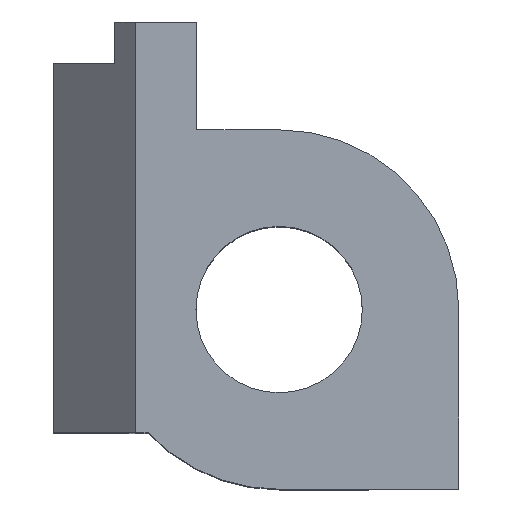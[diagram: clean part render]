
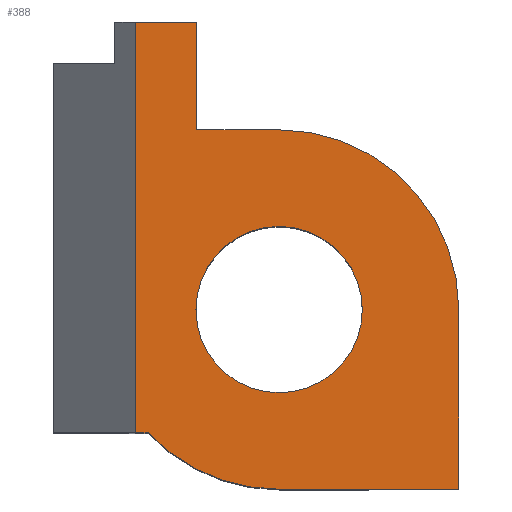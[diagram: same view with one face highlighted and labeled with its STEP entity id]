
A CAD part, top view. The second image highlights one B-rep face of the part: STEP entity #388.
In plain terms, the highlighted planar face has unit normal (0, 0, 1).
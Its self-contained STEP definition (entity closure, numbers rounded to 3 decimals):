
#222=CARTESIAN_POINT('',(-7.,14.,9.9));
#223=VERTEX_POINT('',#222);
#230=CARTESIAN_POINT('',(-4.,14.,9.9));
#231=VERTEX_POINT('',#230);
#232=CARTESIAN_POINT('',(-7.,14.,9.9));
#233=DIRECTION('',(1.0,0.0,0.0));
#234=VECTOR('',#233,3.);
#235=LINE('',#232,#234);
#236=EDGE_CURVE('',#223,#231,#235,.T.);
#293=CARTESIAN_POINT('',(-7.,-6.,9.9));
#294=VERTEX_POINT('',#293);
#301=CARTESIAN_POINT('',(-7.,-6.,9.9));
#302=DIRECTION('',(0.0,1.0,0.0));
#303=VECTOR('',#302,20.);
#304=LINE('',#301,#303);
#305=EDGE_CURVE('',#294,#223,#304,.T.);
#312=CARTESIAN_POINT('',(-9.5,13.0,9.9));
#313=DIRECTION('',(0.0,0.0,1.0));
#314=DIRECTION('',(1.0,0.0,0.0));
#315=AXIS2_PLACEMENT_3D('',#312,#313,#314);
#316=PLANE('',#315);
#317=ORIENTED_EDGE('',*,*,#305,.F.);
#318=CARTESIAN_POINT('',(-6.369,-6.,9.9));
#319=VERTEX_POINT('',#318);
#320=CARTESIAN_POINT('',(-6.369,-6.,9.9));
#321=DIRECTION('',(-1.0,0.0,0.0));
#322=VECTOR('',#321,0.631);
#323=LINE('',#320,#322);
#324=EDGE_CURVE('',#319,#294,#323,.T.);
#325=ORIENTED_EDGE('',*,*,#324,.F.);
#326=CARTESIAN_POINT('',(0.,-8.75,9.9));
#327=VERTEX_POINT('',#326);
#328=CARTESIAN_POINT('',(0.0,0.0,9.9));
#329=DIRECTION('',(0.0,0.0,-1.0));
#330=DIRECTION('',(1.0,0.0,0.0));
#331=AXIS2_PLACEMENT_3D('',#328,#329,#330);
#332=CIRCLE('',#331,8.75);
#333=EDGE_CURVE('',#327,#319,#332,.T.);
#334=ORIENTED_EDGE('',*,*,#333,.F.);
#335=CARTESIAN_POINT('',(8.75,-8.75,9.9));
#336=VERTEX_POINT('',#335);
#337=CARTESIAN_POINT('',(8.75,-8.75,9.9));
#338=DIRECTION('',(-1.0,0.0,0.0));
#339=VECTOR('',#338,8.75);
#340=LINE('',#337,#339);
#341=EDGE_CURVE('',#336,#327,#340,.T.);
#342=ORIENTED_EDGE('',*,*,#341,.F.);
#343=CARTESIAN_POINT('',(8.75,0.,9.9));
#344=VERTEX_POINT('',#343);
#345=CARTESIAN_POINT('',(8.75,0.,9.9));
#346=DIRECTION('',(0.0,-1.0,0.0));
#347=VECTOR('',#346,8.75);
#348=LINE('',#345,#347);
#349=EDGE_CURVE('',#344,#336,#348,.T.);
#350=ORIENTED_EDGE('',*,*,#349,.F.);
#351=CARTESIAN_POINT('',(0.0,8.75,9.9));
#352=VERTEX_POINT('',#351);
#353=CARTESIAN_POINT('',(0.0,0.0,9.9));
#354=DIRECTION('',(0.0,0.0,-1.0));
#355=DIRECTION('',(1.0,0.0,0.0));
#356=AXIS2_PLACEMENT_3D('',#353,#354,#355);
#357=CIRCLE('',#356,8.75);
#358=EDGE_CURVE('',#352,#344,#357,.T.);
#359=ORIENTED_EDGE('',*,*,#358,.F.);
#360=CARTESIAN_POINT('',(-4.,8.75,9.9));
#361=VERTEX_POINT('',#360);
#362=CARTESIAN_POINT('',(-4.,8.75,9.9));
#363=DIRECTION('',(1.0,0.0,0.0));
#364=VECTOR('',#363,4.);
#365=LINE('',#362,#364);
#366=EDGE_CURVE('',#361,#352,#365,.T.);
#367=ORIENTED_EDGE('',*,*,#366,.F.);
#368=CARTESIAN_POINT('',(-4.,14.,9.9));
#369=DIRECTION('',(0.0,-1.0,0.0));
#370=VECTOR('',#369,5.25);
#371=LINE('',#368,#370);
#372=EDGE_CURVE('',#231,#361,#371,.T.);
#373=ORIENTED_EDGE('',*,*,#372,.F.);
#374=ORIENTED_EDGE('',*,*,#236,.F.);
#375=EDGE_LOOP('',(#317,#325,#334,#342,#350,#359,#367,#373,#374));
#376=FACE_OUTER_BOUND('',#375,.T.);
#377=CARTESIAN_POINT('',(4.05,0.,9.9));
#378=VERTEX_POINT('',#377);
#379=CARTESIAN_POINT('',(0.0,0.0,9.9));
#380=DIRECTION('',(0.0,0.0,-1.0));
#381=DIRECTION('',(-1.0,0.0,0.0));
#382=AXIS2_PLACEMENT_3D('',#379,#380,#381);
#383=CIRCLE('',#382,4.05);
#384=EDGE_CURVE('',#378,#378,#383,.T.);
#385=ORIENTED_EDGE('',*,*,#384,.T.);
#386=EDGE_LOOP('',(#385));
#387=FACE_BOUND('',#386,.T.);
#388=ADVANCED_FACE('',(#376,#387),#316,.T.);
